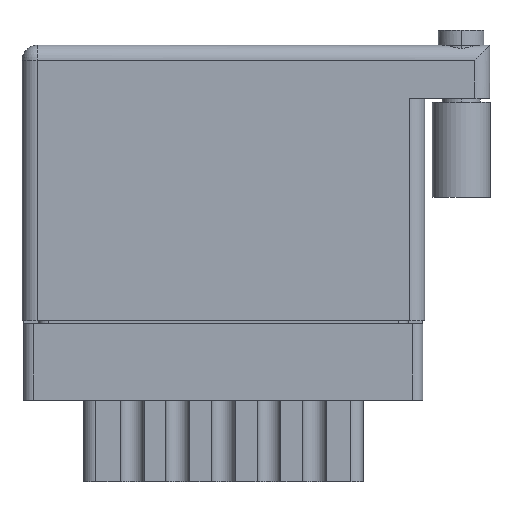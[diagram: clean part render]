
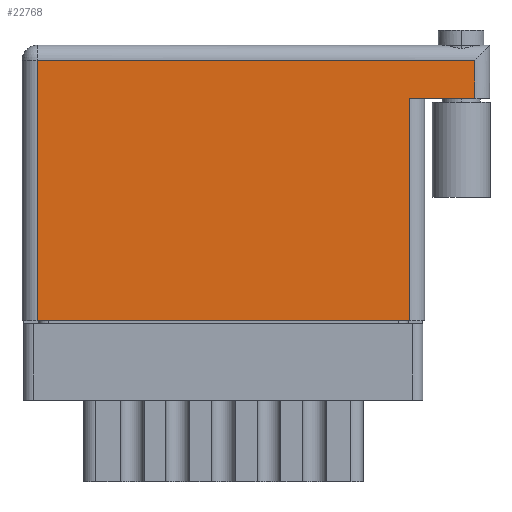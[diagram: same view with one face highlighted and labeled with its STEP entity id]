
A CAD part, front view. The second image highlights one B-rep face of the part: STEP entity #22768.
In plain terms, the highlighted face is planar.
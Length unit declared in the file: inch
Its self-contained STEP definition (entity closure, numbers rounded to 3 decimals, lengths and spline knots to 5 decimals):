
#467 = LINE ( 'NONE', #11625, #23132 ) ;
#670 = PLANE ( 'NONE',  #18245 ) ;
#1204 = EDGE_CURVE ( 'NONE', #9941, #4068, #9727, .T. ) ;
#3101 = ORIENTED_EDGE ( 'NONE', *, *, #1204, .T. ) ;
#3710 = DIRECTION ( 'NONE',  ( 0., 1., 0. ) ) ;
#4068 = VERTEX_POINT ( 'NONE', #10639 ) ;
#4131 = VECTOR ( 'NONE', #13764, 39.37008 ) ;
#4442 = CARTESIAN_POINT ( 'NONE',  ( 0., 0., 0. ) ) ;
#4450 = DIRECTION ( 'NONE',  ( -1., 0., 0. ) ) ;
#4457 = ORIENTED_EDGE ( 'NONE', *, *, #16265, .T. ) ;
#5813 = CARTESIAN_POINT ( 'NONE',  ( 1.489, 0.856, 0. ) ) ;
#6857 = FACE_OUTER_BOUND ( 'NONE', #6863, .T. ) ;
#6863 = EDGE_LOOP ( 'NONE', ( #3101, #16769, #10123, #19276, #4457, #12697 ) ) ;
#8001 = EDGE_CURVE ( 'NONE', #16931, #9941, #9781, .T. ) ;
#9727 = LINE ( 'NONE', #4442, #26085 ) ;
#9781 = LINE ( 'NONE', #25707, #23968 ) ;
#9941 = VERTEX_POINT ( 'NONE', #21897 ) ;
#10123 = ORIENTED_EDGE ( 'NONE', *, *, #16387, .F. ) ;
#10508 = CARTESIAN_POINT ( 'NONE',  ( 1.275, 0.731, 0. ) ) ;
#10538 = LINE ( 'NONE', #20967, #25987 ) ;
#10639 = CARTESIAN_POINT ( 'NONE',  ( 1.275, 0., 0. ) ) ;
#11625 = CARTESIAN_POINT ( 'NONE',  ( 1.539, 0.731, 0. ) ) ;
#12070 = EDGE_CURVE ( 'NONE', #20233, #22076, #23083, .T. ) ;
#12697 = ORIENTED_EDGE ( 'NONE', *, *, #8001, .T. ) ;
#12893 = CARTESIAN_POINT ( 'NONE',  ( 0., 0.906, 0. ) ) ;
#13221 = DIRECTION ( 'NONE',  ( -1., 0., 0. ) ) ;
#13764 = DIRECTION ( 'NONE',  ( 0., 1., 0. ) ) ;
#16265 = EDGE_CURVE ( 'NONE', #22076, #16931, #10538, .T. ) ;
#16387 = EDGE_CURVE ( 'NONE', #20233, #18774, #467, .T. ) ;
#16558 = CARTESIAN_POINT ( 'NONE',  ( 0.05, 0.856, 0. ) ) ;
#16769 = ORIENTED_EDGE ( 'NONE', *, *, #18114, .T. ) ;
#16931 = VERTEX_POINT ( 'NONE', #16558 ) ;
#18114 = EDGE_CURVE ( 'NONE', #4068, #18774, #23065, .T. ) ;
#18245 = AXIS2_PLACEMENT_3D ( 'NONE', #12893, #20584, #4450 ) ;
#18774 = VERTEX_POINT ( 'NONE', #10508 ) ;
#19276 = ORIENTED_EDGE ( 'NONE', *, *, #12070, .T. ) ;
#19672 = CARTESIAN_POINT ( 'NONE',  ( 1.489, 0.906, 0. ) ) ;
#20233 = VERTEX_POINT ( 'NONE', #20719 ) ;
#20394 = DIRECTION ( 'NONE',  ( 1., 0., 0. ) ) ;
#20584 = DIRECTION ( 'NONE',  ( 0., 0., -1. ) ) ;
#20719 = CARTESIAN_POINT ( 'NONE',  ( 1.489, 0.731, 0. ) ) ;
#20967 = CARTESIAN_POINT ( 'NONE',  ( 0., 0.856, 0. ) ) ;
#21354 = CARTESIAN_POINT ( 'NONE',  ( 1.275, 0.731, 0. ) ) ;
#21744 = DIRECTION ( 'NONE',  ( 0., -1., 0. ) ) ;
#21897 = CARTESIAN_POINT ( 'NONE',  ( 0.05, 0., 0. ) ) ;
#22076 = VERTEX_POINT ( 'NONE', #5813 ) ;
#22154 = VECTOR ( 'NONE', #3710, 39.37008 ) ;
#22768 = ADVANCED_FACE ( 'NONE', ( #6857 ), #670, .F. ) ;
#23065 = LINE ( 'NONE', #21354, #4131 ) ;
#23083 = LINE ( 'NONE', #19672, #22154 ) ;
#23132 = VECTOR ( 'NONE', #23356, 39.37008 ) ;
#23356 = DIRECTION ( 'NONE',  ( -1., 0., 0. ) ) ;
#23968 = VECTOR ( 'NONE', #21744, 39.37008 ) ;
#25707 = CARTESIAN_POINT ( 'NONE',  ( 0.05, 0., 0. ) ) ;
#25987 = VECTOR ( 'NONE', #13221, 39.37008 ) ;
#26085 = VECTOR ( 'NONE', #20394, 39.37008 ) ;
